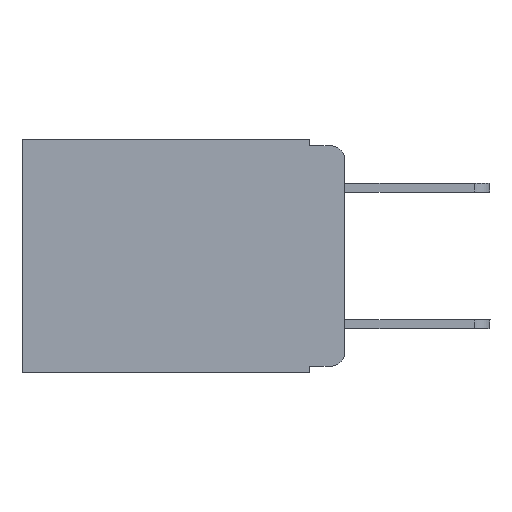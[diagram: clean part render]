
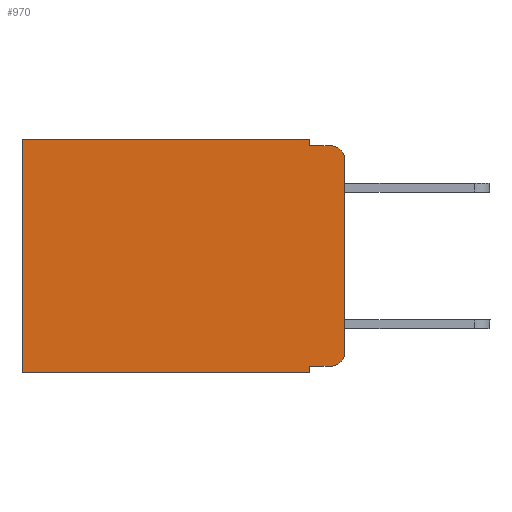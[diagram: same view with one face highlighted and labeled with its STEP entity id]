
A CAD part, left-side view. The second image highlights one B-rep face of the part: STEP entity #970.
In plain terms, the highlighted planar face has unit normal (-1, 0, 0).
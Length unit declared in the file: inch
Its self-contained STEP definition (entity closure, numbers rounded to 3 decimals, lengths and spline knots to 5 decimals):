
#217 = VECTOR ( 'NONE', #864, 39.37008 ) ;
#384 = VECTOR ( 'NONE', #10359, 39.37008 ) ;
#430 = CARTESIAN_POINT ( 'NONE',  ( 0.298, 0.051, -0.333 ) ) ;
#464 = ORIENTED_EDGE ( 'NONE', *, *, #9446, .T. ) ;
#506 = VECTOR ( 'NONE', #7356, 39.37008 ) ;
#574 = VERTEX_POINT ( 'NONE', #10502 ) ;
#603 = VECTOR ( 'NONE', #9957, 39.37008 ) ;
#641 = LINE ( 'NONE', #7296, #506 ) ;
#864 = DIRECTION ( 'NONE',  ( 0., 1., 0. ) ) ;
#952 = EDGE_CURVE ( 'NONE', #9054, #7239, #3982, .T. ) ;
#970 = ADVANCED_FACE ( 'NONE', ( #3867 ), #6876, .F. ) ;
#984 = CARTESIAN_POINT ( 'NONE',  ( 0.298, 0.051, 0. ) ) ;
#1046 = CARTESIAN_POINT ( 'NONE',  ( 0.298, 0.051, -0.01 ) ) ;
#1062 = DIRECTION ( 'NONE',  ( 0., 0., -1. ) ) ;
#1095 = CARTESIAN_POINT ( 'NONE',  ( 0.298, 0.02, -0.03 ) ) ;
#1130 = DIRECTION ( 'NONE',  ( 0., 0., -1. ) ) ;
#1306 = VERTEX_POINT ( 'NONE', #8136 ) ;
#1523 = VERTEX_POINT ( 'NONE', #6017 ) ;
#1756 = CARTESIAN_POINT ( 'NONE',  ( 0.298, 0., 0. ) ) ;
#1856 = VERTEX_POINT ( 'NONE', #5096 ) ;
#1935 = EDGE_CURVE ( 'NONE', #1856, #1523, #7998, .T. ) ;
#1971 = EDGE_CURVE ( 'NONE', #1856, #574, #8362, .T. ) ;
#2147 = VECTOR ( 'NONE', #2586, 39.37008 ) ;
#2213 = DIRECTION ( 'NONE',  ( 0., 0., -1. ) ) ;
#2216 = CARTESIAN_POINT ( 'NONE',  ( 0.298, 0., -0.313 ) ) ;
#2260 = AXIS2_PLACEMENT_3D ( 'NONE', #7721, #2755, #9457 ) ;
#2548 = AXIS2_PLACEMENT_3D ( 'NONE', #1095, #2787, #1130 ) ;
#2586 = DIRECTION ( 'NONE',  ( 0., 0., -1. ) ) ;
#2646 = LINE ( 'NONE', #1046, #384 ) ;
#2693 = VERTEX_POINT ( 'NONE', #8565 ) ;
#2755 = DIRECTION ( 'NONE',  ( 1., 0., 0. ) ) ;
#2787 = DIRECTION ( 'NONE',  ( -1., 0., 0. ) ) ;
#2975 = EDGE_CURVE ( 'NONE', #1306, #4274, #641, .T. ) ;
#3251 = ORIENTED_EDGE ( 'NONE', *, *, #2975, .T. ) ;
#3416 = CARTESIAN_POINT ( 'NONE',  ( 0.298, 0., 0. ) ) ;
#3485 = ORIENTED_EDGE ( 'NONE', *, *, #10910, .T. ) ;
#3867 = FACE_OUTER_BOUND ( 'NONE', #7343, .T. ) ;
#3944 = CARTESIAN_POINT ( 'NONE',  ( 0.298, 0.02, -0.313 ) ) ;
#3982 = LINE ( 'NONE', #1756, #10514 ) ;
#4274 = VERTEX_POINT ( 'NONE', #6299 ) ;
#4404 = EDGE_CURVE ( 'NONE', #10588, #8636, #4964, .T. ) ;
#4964 = LINE ( 'NONE', #5561, #603 ) ;
#4974 = CARTESIAN_POINT ( 'NONE',  ( 0.298, 0., -0.03 ) ) ;
#5041 = ORIENTED_EDGE ( 'NONE', *, *, #952, .F. ) ;
#5096 = CARTESIAN_POINT ( 'NONE',  ( 0.298, 0.051, -0.333 ) ) ;
#5561 = CARTESIAN_POINT ( 'NONE',  ( 0.298, 0.051, 0. ) ) ;
#5636 = LINE ( 'NONE', #3416, #217 ) ;
#5894 = VECTOR ( 'NONE', #8107, 39.37008 ) ;
#6017 = CARTESIAN_POINT ( 'NONE',  ( 0.298, 0.02, -0.333 ) ) ;
#6299 = CARTESIAN_POINT ( 'NONE',  ( 0.298, 0.473, -0.343 ) ) ;
#6581 = CIRCLE ( 'NONE', #7592, 0.02 ) ;
#6876 = PLANE ( 'NONE',  #2260 ) ;
#7157 = CARTESIAN_POINT ( 'NONE',  ( 0.298, 0., -0.343 ) ) ;
#7239 = VERTEX_POINT ( 'NONE', #2216 ) ;
#7253 = ORIENTED_EDGE ( 'NONE', *, *, #10033, .F. ) ;
#7296 = CARTESIAN_POINT ( 'NONE',  ( 0.298, 0.473, 0. ) ) ;
#7343 = EDGE_LOOP ( 'NONE', ( #5041, #3485, #10280, #9426, #7523, #3251, #7253, #8848, #9512, #464 ) ) ;
#7356 = DIRECTION ( 'NONE',  ( 0., 0., -1. ) ) ;
#7523 = ORIENTED_EDGE ( 'NONE', *, *, #9648, .T. ) ;
#7592 = AXIS2_PLACEMENT_3D ( 'NONE', #3944, #10733, #2213 ) ;
#7632 = CARTESIAN_POINT ( 'NONE',  ( 0.298, 0.051, 0. ) ) ;
#7657 = CIRCLE ( 'NONE', #2548, 0.02 ) ;
#7721 = CARTESIAN_POINT ( 'NONE',  ( 0.298, 0., 0. ) ) ;
#7844 = CARTESIAN_POINT ( 'NONE',  ( 0.298, 0.051, -0.01 ) ) ;
#7998 = LINE ( 'NONE', #430, #11010 ) ;
#8107 = DIRECTION ( 'NONE',  ( 0., 1., 0. ) ) ;
#8136 = CARTESIAN_POINT ( 'NONE',  ( 0.298, 0.473, 0. ) ) ;
#8362 = LINE ( 'NONE', #7632, #2147 ) ;
#8565 = CARTESIAN_POINT ( 'NONE',  ( 0.298, 0.02, -0.01 ) ) ;
#8636 = VERTEX_POINT ( 'NONE', #7844 ) ;
#8848 = ORIENTED_EDGE ( 'NONE', *, *, #1971, .F. ) ;
#9054 = VERTEX_POINT ( 'NONE', #4974 ) ;
#9149 = EDGE_CURVE ( 'NONE', #8636, #2693, #2646, .T. ) ;
#9426 = ORIENTED_EDGE ( 'NONE', *, *, #4404, .F. ) ;
#9446 = EDGE_CURVE ( 'NONE', #1523, #7239, #6581, .T. ) ;
#9457 = DIRECTION ( 'NONE',  ( 0., 0., -1. ) ) ;
#9512 = ORIENTED_EDGE ( 'NONE', *, *, #1935, .T. ) ;
#9648 = EDGE_CURVE ( 'NONE', #10588, #1306, #5636, .T. ) ;
#9957 = DIRECTION ( 'NONE',  ( 0., 0., -1. ) ) ;
#10033 = EDGE_CURVE ( 'NONE', #574, #4274, #10951, .T. ) ;
#10165 = DIRECTION ( 'NONE',  ( 0., -1., 0. ) ) ;
#10280 = ORIENTED_EDGE ( 'NONE', *, *, #9149, .F. ) ;
#10359 = DIRECTION ( 'NONE',  ( 0., -1., 0. ) ) ;
#10502 = CARTESIAN_POINT ( 'NONE',  ( 0.298, 0.051, -0.343 ) ) ;
#10514 = VECTOR ( 'NONE', #1062, 39.37008 ) ;
#10588 = VERTEX_POINT ( 'NONE', #984 ) ;
#10733 = DIRECTION ( 'NONE',  ( -1., 0., 0. ) ) ;
#10910 = EDGE_CURVE ( 'NONE', #9054, #2693, #7657, .T. ) ;
#10951 = LINE ( 'NONE', #7157, #5894 ) ;
#11010 = VECTOR ( 'NONE', #10165, 39.37008 ) ;
